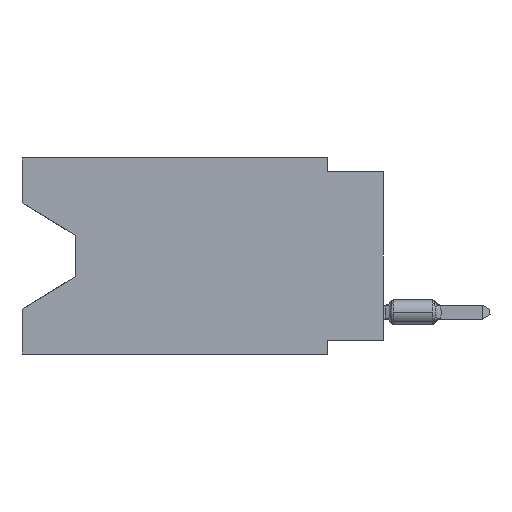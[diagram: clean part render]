
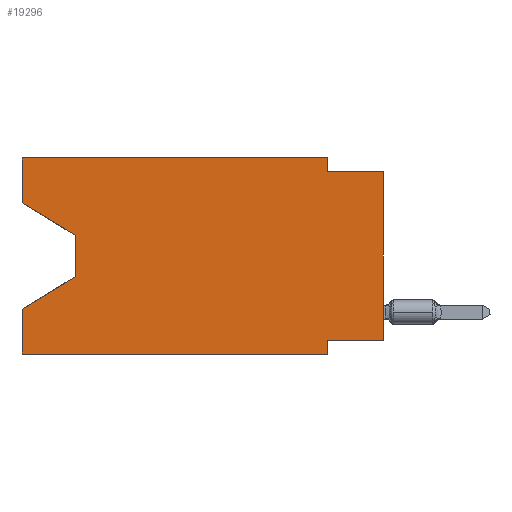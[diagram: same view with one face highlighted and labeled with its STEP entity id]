
A CAD part, left-side view. The second image highlights one B-rep face of the part: STEP entity #19296.
In plain terms, the highlighted planar face has unit normal (-1, 0, 0).
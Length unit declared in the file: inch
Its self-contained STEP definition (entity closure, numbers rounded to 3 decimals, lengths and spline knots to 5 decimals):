
#282 = VERTEX_POINT ( 'NONE', #24508 ) ;
#350 = VECTOR ( 'NONE', #21775, 39.37008 ) ;
#464 = VECTOR ( 'NONE', #4720, 39.37008 ) ;
#760 = EDGE_CURVE ( 'NONE', #11168, #14651, #10333, .T. ) ;
#829 = ORIENTED_EDGE ( 'NONE', *, *, #4171, .F. ) ;
#1264 = ORIENTED_EDGE ( 'NONE', *, *, #5124, .F. ) ;
#2283 = CARTESIAN_POINT ( 'NONE',  ( 0., 0.1, 0. ) ) ;
#2554 = ORIENTED_EDGE ( 'NONE', *, *, #14782, .T. ) ;
#2877 = LINE ( 'NONE', #10842, #464 ) ;
#3372 = CARTESIAN_POINT ( 'NONE',  ( 0., 0.645, -0.35 ) ) ;
#3528 = CARTESIAN_POINT ( 'NONE',  ( 0., 0.645, -0.08025 ) ) ;
#3665 = LINE ( 'NONE', #5505, #8230 ) ;
#4171 = EDGE_CURVE ( 'NONE', #12188, #282, #22201, .T. ) ;
#4272 = CARTESIAN_POINT ( 'NONE',  ( 0., 0.645, 0. ) ) ;
#4310 = VERTEX_POINT ( 'NONE', #5179 ) ;
#4369 = VERTEX_POINT ( 'NONE', #7783 ) ;
#4645 = ORIENTED_EDGE ( 'NONE', *, *, #20953, .T. ) ;
#4720 = DIRECTION ( 'NONE',  ( 0., 0.855, -0.519 ) ) ;
#5090 = LINE ( 'NONE', #21166, #23835 ) ;
#5124 = EDGE_CURVE ( 'NONE', #4369, #4310, #3665, .T. ) ;
#5179 = CARTESIAN_POINT ( 'NONE',  ( 0., 0.1, -0.35 ) ) ;
#5505 = CARTESIAN_POINT ( 'NONE',  ( 0., 0.1, -0.35 ) ) ;
#5593 = CARTESIAN_POINT ( 'NONE',  ( 0., 0.1, -0.025 ) ) ;
#5631 = ORIENTED_EDGE ( 'NONE', *, *, #8553, .F. ) ;
#7412 = VERTEX_POINT ( 'NONE', #3528 ) ;
#7783 = CARTESIAN_POINT ( 'NONE',  ( 0., 0.1, -0.325 ) ) ;
#7899 = VECTOR ( 'NONE', #19849, 39.37008 ) ;
#8028 = PLANE ( 'NONE',  #10777 ) ;
#8230 = VECTOR ( 'NONE', #18018, 39.37008 ) ;
#8397 = DIRECTION ( 'NONE',  ( 0., 0., -1. ) ) ;
#8432 = VECTOR ( 'NONE', #22708, 39.37008 ) ;
#8502 = CARTESIAN_POINT ( 'NONE',  ( 0., 0.645, 0. ) ) ;
#8553 = EDGE_CURVE ( 'NONE', #13510, #11168, #20650, .T. ) ;
#8685 = LINE ( 'NONE', #16666, #8432 ) ;
#8939 = VERTEX_POINT ( 'NONE', #9507 ) ;
#9160 = VECTOR ( 'NONE', #23601, 39.37008 ) ;
#9380 = DIRECTION ( 'NONE',  ( 0., -1., 0. ) ) ;
#9507 = CARTESIAN_POINT ( 'NONE',  ( 0., 0.55, -0.212 ) ) ;
#10258 = CARTESIAN_POINT ( 'NONE',  ( 0., 0., 0. ) ) ;
#10333 = LINE ( 'NONE', #18326, #20705 ) ;
#10759 = LINE ( 'NONE', #15481, #350 ) ;
#10777 = AXIS2_PLACEMENT_3D ( 'NONE', #21902, #20187, #14019 ) ;
#10842 = CARTESIAN_POINT ( 'NONE',  ( 0., 0.55, -0.212 ) ) ;
#11073 = CARTESIAN_POINT ( 'NONE',  ( 0., 0., -0.025 ) ) ;
#11080 = DIRECTION ( 'NONE',  ( 0., -1., 0. ) ) ;
#11168 = VERTEX_POINT ( 'NONE', #2283 ) ;
#11465 = EDGE_CURVE ( 'NONE', #19565, #8939, #10759, .T. ) ;
#11846 = ORIENTED_EDGE ( 'NONE', *, *, #11465, .T. ) ;
#12188 = VERTEX_POINT ( 'NONE', #12678 ) ;
#12237 = DIRECTION ( 'NONE',  ( 0., 0., 1. ) ) ;
#12348 = LINE ( 'NONE', #10258, #7899 ) ;
#12678 = CARTESIAN_POINT ( 'NONE',  ( 0., 0.645, -0.35 ) ) ;
#12958 = ORIENTED_EDGE ( 'NONE', *, *, #20229, .T. ) ;
#13510 = VERTEX_POINT ( 'NONE', #8502 ) ;
#13940 = VERTEX_POINT ( 'NONE', #24837 ) ;
#13977 = VERTEX_POINT ( 'NONE', #11073 ) ;
#13987 = EDGE_CURVE ( 'NONE', #12188, #4310, #23261, .T. ) ;
#14019 = DIRECTION ( 'NONE',  ( 0., 0., -1. ) ) ;
#14538 = VECTOR ( 'NONE', #9380, 39.37008 ) ;
#14555 = ORIENTED_EDGE ( 'NONE', *, *, #760, .F. ) ;
#14651 = VERTEX_POINT ( 'NONE', #5593 ) ;
#14782 = EDGE_CURVE ( 'NONE', #13940, #13977, #12348, .T. ) ;
#15481 = CARTESIAN_POINT ( 'NONE',  ( 0., 0.55, -0.138 ) ) ;
#15723 = FACE_OUTER_BOUND ( 'NONE', #19414, .T. ) ;
#16666 = CARTESIAN_POINT ( 'NONE',  ( 0., 0.645, -0.08025 ) ) ;
#16713 = CARTESIAN_POINT ( 'NONE',  ( 0., 0.645, 0. ) ) ;
#17508 = EDGE_CURVE ( 'NONE', #14651, #13977, #5090, .T. ) ;
#17931 = ORIENTED_EDGE ( 'NONE', *, *, #22957, .F. ) ;
#18018 = DIRECTION ( 'NONE',  ( 0., 0., -1. ) ) ;
#18286 = DIRECTION ( 'NONE',  ( 0., -1., 0. ) ) ;
#18326 = CARTESIAN_POINT ( 'NONE',  ( 0., 0.1, 0. ) ) ;
#18466 = ORIENTED_EDGE ( 'NONE', *, *, #17508, .F. ) ;
#19296 = ADVANCED_FACE ( 'NONE', ( #15723 ), #8028, .F. ) ;
#19414 = EDGE_LOOP ( 'NONE', ( #12958, #11846, #4645, #829, #23860, #1264, #24444, #2554, #18466, #14555, #5631, #17931 ) ) ;
#19565 = VERTEX_POINT ( 'NONE', #21482 ) ;
#19612 = LINE ( 'NONE', #23419, #21277 ) ;
#19806 = LINE ( 'NONE', #21505, #9160 ) ;
#19849 = DIRECTION ( 'NONE',  ( 0., 0., 1. ) ) ;
#20187 = DIRECTION ( 'NONE',  ( 1., 0., 0. ) ) ;
#20229 = EDGE_CURVE ( 'NONE', #7412, #19565, #8685, .T. ) ;
#20650 = LINE ( 'NONE', #16713, #25398 ) ;
#20705 = VECTOR ( 'NONE', #8397, 39.37008 ) ;
#20953 = EDGE_CURVE ( 'NONE', #8939, #282, #2877, .T. ) ;
#21166 = CARTESIAN_POINT ( 'NONE',  ( 0., 0., -0.025 ) ) ;
#21277 = VECTOR ( 'NONE', #25503, 39.37008 ) ;
#21482 = CARTESIAN_POINT ( 'NONE',  ( 0., 0.55, -0.138 ) ) ;
#21505 = CARTESIAN_POINT ( 'NONE',  ( 0., 0.645, 0. ) ) ;
#21775 = DIRECTION ( 'NONE',  ( 0., 0., -1. ) ) ;
#21902 = CARTESIAN_POINT ( 'NONE',  ( 0., 0.645, 0. ) ) ;
#22188 = EDGE_CURVE ( 'NONE', #13940, #4369, #19612, .T. ) ;
#22201 = LINE ( 'NONE', #4272, #25085 ) ;
#22708 = DIRECTION ( 'NONE',  ( 0., -0.855, -0.519 ) ) ;
#22957 = EDGE_CURVE ( 'NONE', #7412, #13510, #19806, .T. ) ;
#23261 = LINE ( 'NONE', #3372, #14538 ) ;
#23419 = CARTESIAN_POINT ( 'NONE',  ( 0., 0., -0.325 ) ) ;
#23601 = DIRECTION ( 'NONE',  ( 0., 0., 1. ) ) ;
#23835 = VECTOR ( 'NONE', #11080, 39.37008 ) ;
#23860 = ORIENTED_EDGE ( 'NONE', *, *, #13987, .T. ) ;
#24444 = ORIENTED_EDGE ( 'NONE', *, *, #22188, .F. ) ;
#24508 = CARTESIAN_POINT ( 'NONE',  ( 0., 0.645, -0.26975 ) ) ;
#24837 = CARTESIAN_POINT ( 'NONE',  ( 0., 0., -0.325 ) ) ;
#25085 = VECTOR ( 'NONE', #12237, 39.37008 ) ;
#25398 = VECTOR ( 'NONE', #18286, 39.37008 ) ;
#25503 = DIRECTION ( 'NONE',  ( 0., 1., 0. ) ) ;
